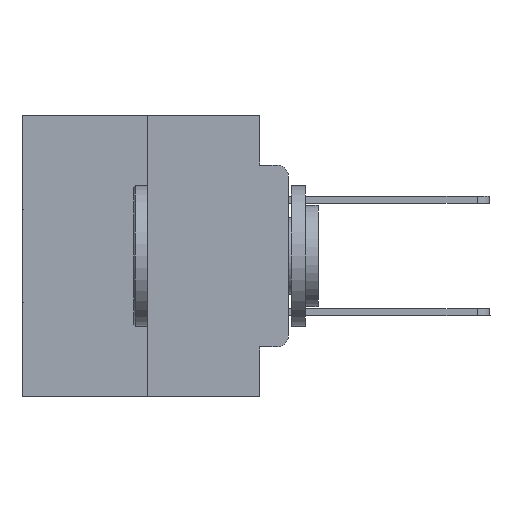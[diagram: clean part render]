
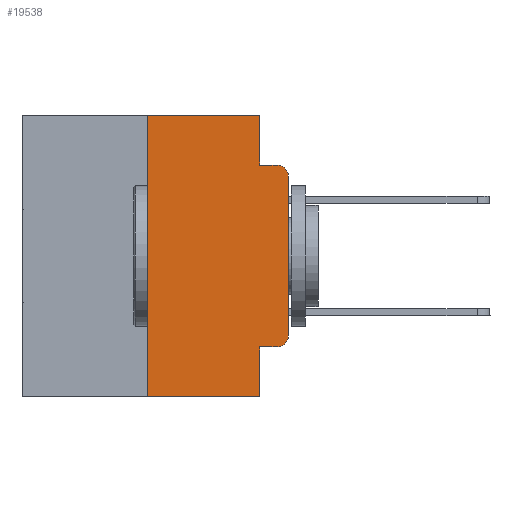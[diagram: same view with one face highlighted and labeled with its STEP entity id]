
A CAD part, left-side view. The second image highlights one B-rep face of the part: STEP entity #19538.
In plain terms, the highlighted planar face has unit normal (-1, 0, 0).
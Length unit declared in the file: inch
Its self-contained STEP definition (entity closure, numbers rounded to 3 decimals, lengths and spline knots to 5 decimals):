
#25 = CARTESIAN_POINT ( 'NONE',  ( 0., 0.02, -0.4115 ) ) ;
#45 = ORIENTED_EDGE ( 'NONE', *, *, #28361, .T. ) ;
#878 = ORIENTED_EDGE ( 'NONE', *, *, #11525, .F. ) ;
#965 = DIRECTION ( 'NONE',  ( 0., 0., -1. ) ) ;
#1285 = VECTOR ( 'NONE', #2535, 39.37008 ) ;
#1333 = EDGE_CURVE ( 'NONE', #14549, #2553, #9352, .T. ) ;
#1553 = VECTOR ( 'NONE', #27647, 39.37008 ) ;
#2049 = CARTESIAN_POINT ( 'NONE',  ( 0., 0.051, -0.5 ) ) ;
#2205 = CARTESIAN_POINT ( 'NONE',  ( 0., 0.25, -0.5 ) ) ;
#2535 = DIRECTION ( 'NONE',  ( 0., 0., 1. ) ) ;
#2553 = VERTEX_POINT ( 'NONE', #24992 ) ;
#2671 = AXIS2_PLACEMENT_3D ( 'NONE', #22919, #13711, #16554 ) ;
#2762 = EDGE_CURVE ( 'NONE', #5053, #19032, #12871, .T. ) ;
#2812 = LINE ( 'NONE', #6258, #8952 ) ;
#3302 = LINE ( 'NONE', #26499, #27198 ) ;
#3601 = VECTOR ( 'NONE', #21057, 39.37008 ) ;
#3695 = CARTESIAN_POINT ( 'NONE',  ( 0., 0.051, -0.0885 ) ) ;
#3760 = DIRECTION ( 'NONE',  ( 0., 0., -1. ) ) ;
#4232 = ORIENTED_EDGE ( 'NONE', *, *, #10961, .T. ) ;
#5053 = VERTEX_POINT ( 'NONE', #2205 ) ;
#5398 = LINE ( 'NONE', #14048, #3601 ) ;
#5445 = DIRECTION ( 'NONE',  ( 0., 0., -1. ) ) ;
#6258 = CARTESIAN_POINT ( 'NONE',  ( 0., 0.051, 0. ) ) ;
#6562 = DIRECTION ( 'NONE',  ( 0., -1., 0. ) ) ;
#6790 = ORIENTED_EDGE ( 'NONE', *, *, #2762, .F. ) ;
#7451 = ORIENTED_EDGE ( 'NONE', *, *, #1333, .T. ) ;
#7945 = PLANE ( 'NONE',  #12249 ) ;
#8952 = VECTOR ( 'NONE', #3760, 39.37008 ) ;
#9001 = EDGE_CURVE ( 'NONE', #23120, #23702, #26941, .T. ) ;
#9352 = CIRCLE ( 'NONE', #2671, 0.02 ) ;
#9772 = FACE_OUTER_BOUND ( 'NONE', #29273, .T. ) ;
#9896 = ORIENTED_EDGE ( 'NONE', *, *, #23698, .F. ) ;
#10302 = CARTESIAN_POINT ( 'NONE',  ( 0., 0.473, 0. ) ) ;
#10816 = DIRECTION ( 'NONE',  ( -1., 0., 0. ) ) ;
#10961 = EDGE_CURVE ( 'NONE', #29739, #14549, #3302, .T. ) ;
#11231 = CARTESIAN_POINT ( 'NONE',  ( 0., 0.051, -0.4115 ) ) ;
#11525 = EDGE_CURVE ( 'NONE', #23702, #2553, #28576, .T. ) ;
#12249 = AXIS2_PLACEMENT_3D ( 'NONE', #10302, #26492, #5445 ) ;
#12871 = LINE ( 'NONE', #21191, #1285 ) ;
#13711 = DIRECTION ( 'NONE',  ( -1., 0., 0. ) ) ;
#13914 = LINE ( 'NONE', #29730, #24013 ) ;
#14048 = CARTESIAN_POINT ( 'NONE',  ( 0., 0.051, -0.4115 ) ) ;
#14492 = VECTOR ( 'NONE', #24425, 39.37008 ) ;
#14549 = VERTEX_POINT ( 'NONE', #15382 ) ;
#15068 = ORIENTED_EDGE ( 'NONE', *, *, #9001, .F. ) ;
#15382 = CARTESIAN_POINT ( 'NONE',  ( 0., 0., -0.1085 ) ) ;
#15912 = CIRCLE ( 'NONE', #23396, 0.02 ) ;
#16387 = EDGE_CURVE ( 'NONE', #5053, #23083, #17864, .T. ) ;
#16533 = ORIENTED_EDGE ( 'NONE', *, *, #20872, .F. ) ;
#16554 = DIRECTION ( 'NONE',  ( 0., 0., -1. ) ) ;
#17844 = VERTEX_POINT ( 'NONE', #25 ) ;
#17864 = LINE ( 'NONE', #20582, #1553 ) ;
#18296 = CARTESIAN_POINT ( 'NONE',  ( 0., 0.25, 0. ) ) ;
#19032 = VERTEX_POINT ( 'NONE', #18296 ) ;
#19538 = ADVANCED_FACE ( 'NONE', ( #9772 ), #7945, .F. ) ;
#20582 = CARTESIAN_POINT ( 'NONE',  ( 0., 0.473, -0.5 ) ) ;
#20627 = ORIENTED_EDGE ( 'NONE', *, *, #16387, .T. ) ;
#20872 = EDGE_CURVE ( 'NONE', #29465, #23083, #2812, .T. ) ;
#21057 = DIRECTION ( 'NONE',  ( 0., -1., 0. ) ) ;
#21191 = CARTESIAN_POINT ( 'NONE',  ( 0., 0.25, 0. ) ) ;
#21379 = CARTESIAN_POINT ( 'NONE',  ( 0., 0., -0.3915 ) ) ;
#21833 = CARTESIAN_POINT ( 'NONE',  ( 0., 0.051, 0. ) ) ;
#22356 = CARTESIAN_POINT ( 'NONE',  ( 0., 0.02, -0.3915 ) ) ;
#22778 = CARTESIAN_POINT ( 'NONE',  ( 0., 0.051, -0.0885 ) ) ;
#22869 = ORIENTED_EDGE ( 'NONE', *, *, #28283, .T. ) ;
#22919 = CARTESIAN_POINT ( 'NONE',  ( 0., 0.02, -0.1085 ) ) ;
#23083 = VERTEX_POINT ( 'NONE', #2049 ) ;
#23120 = VERTEX_POINT ( 'NONE', #29966 ) ;
#23396 = AXIS2_PLACEMENT_3D ( 'NONE', #22356, #10816, #27013 ) ;
#23698 = EDGE_CURVE ( 'NONE', #19032, #23120, #13914, .T. ) ;
#23702 = VERTEX_POINT ( 'NONE', #22778 ) ;
#24013 = VECTOR ( 'NONE', #6562, 39.37008 ) ;
#24425 = DIRECTION ( 'NONE',  ( 0., -1., 0. ) ) ;
#24992 = CARTESIAN_POINT ( 'NONE',  ( 0., 0.02, -0.0885 ) ) ;
#26492 = DIRECTION ( 'NONE',  ( 1., 0., 0. ) ) ;
#26499 = CARTESIAN_POINT ( 'NONE',  ( 0., 0., 0. ) ) ;
#26700 = DIRECTION ( 'NONE',  ( 0., 0., 1. ) ) ;
#26941 = LINE ( 'NONE', #21833, #27657 ) ;
#27013 = DIRECTION ( 'NONE',  ( 0., 0., -1. ) ) ;
#27198 = VECTOR ( 'NONE', #26700, 39.37008 ) ;
#27647 = DIRECTION ( 'NONE',  ( 0., -1., 0. ) ) ;
#27657 = VECTOR ( 'NONE', #965, 39.37008 ) ;
#28283 = EDGE_CURVE ( 'NONE', #17844, #29739, #15912, .T. ) ;
#28361 = EDGE_CURVE ( 'NONE', #29465, #17844, #5398, .T. ) ;
#28576 = LINE ( 'NONE', #3695, #14492 ) ;
#29273 = EDGE_LOOP ( 'NONE', ( #4232, #7451, #878, #15068, #9896, #6790, #20627, #16533, #45, #22869 ) ) ;
#29465 = VERTEX_POINT ( 'NONE', #11231 ) ;
#29730 = CARTESIAN_POINT ( 'NONE',  ( 0., 0.473, 0. ) ) ;
#29739 = VERTEX_POINT ( 'NONE', #21379 ) ;
#29966 = CARTESIAN_POINT ( 'NONE',  ( 0., 0.051, 0. ) ) ;
